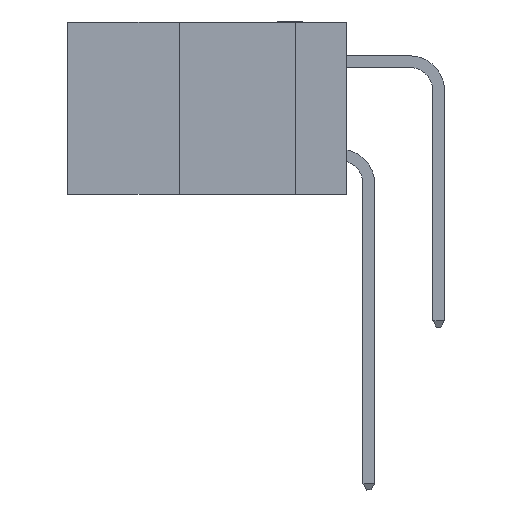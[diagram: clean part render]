
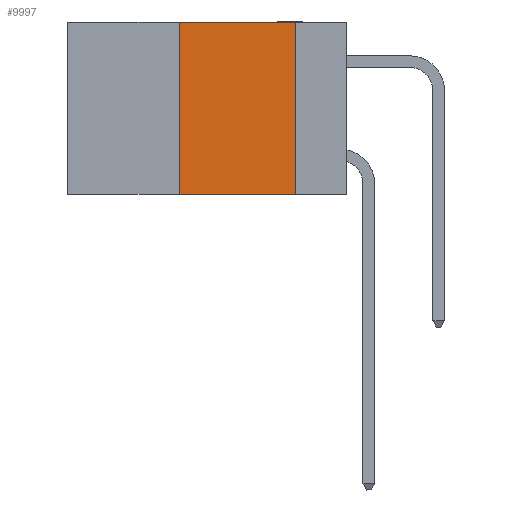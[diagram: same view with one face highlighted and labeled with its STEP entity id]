
A CAD part, left-side view. The second image highlights one B-rep face of the part: STEP entity #9997.
In plain terms, the highlighted planar face has unit normal (-1, 0, 0).
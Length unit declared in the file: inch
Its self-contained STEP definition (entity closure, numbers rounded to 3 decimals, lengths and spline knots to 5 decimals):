
#238 = FACE_OUTER_BOUND ( 'NONE', #1158, .T. ) ;
#518 = LINE ( 'NONE', #21421, #9261 ) ;
#585 = PLANE ( 'NONE',  #2373 ) ;
#899 = VECTOR ( 'NONE', #1618, 39.37008 ) ;
#1158 = EDGE_LOOP ( 'NONE', ( #18078, #10498, #21211, #17680 ) ) ;
#1618 = DIRECTION ( 'NONE',  ( 0., -1., 0. ) ) ;
#2373 = AXIS2_PLACEMENT_3D ( 'NONE', #12823, #14560, #4169 ) ;
#3454 = CARTESIAN_POINT ( 'NONE',  ( 0., 0.11, -0.37 ) ) ;
#3649 = VECTOR ( 'NONE', #14049, 39.37008 ) ;
#4169 = DIRECTION ( 'NONE',  ( 0., 0., -1. ) ) ;
#7463 = EDGE_CURVE ( 'NONE', #20679, #8522, #8081, .T. ) ;
#8081 = LINE ( 'NONE', #21353, #21289 ) ;
#8522 = VERTEX_POINT ( 'NONE', #3454 ) ;
#9073 = VERTEX_POINT ( 'NONE', #15743 ) ;
#9261 = VECTOR ( 'NONE', #11274, 39.37008 ) ;
#9997 = ADVANCED_FACE ( 'NONE', ( #238 ), #585, .F. ) ;
#10498 = ORIENTED_EDGE ( 'NONE', *, *, #18647, .F. ) ;
#11274 = DIRECTION ( 'NONE',  ( 0., 0., -1. ) ) ;
#11620 = VERTEX_POINT ( 'NONE', #16867 ) ;
#12285 = CARTESIAN_POINT ( 'NONE',  ( 0., 0.36, 0. ) ) ;
#12823 = CARTESIAN_POINT ( 'NONE',  ( 0., 0.6, 0. ) ) ;
#12903 = LINE ( 'NONE', #12285, #3649 ) ;
#14049 = DIRECTION ( 'NONE',  ( 0., 0., 1. ) ) ;
#14560 = DIRECTION ( 'NONE',  ( 1., 0., 0. ) ) ;
#14611 = DIRECTION ( 'NONE',  ( 0., -1., 0. ) ) ;
#14820 = LINE ( 'NONE', #22279, #899 ) ;
#15113 = EDGE_CURVE ( 'NONE', #11620, #8522, #518, .T. ) ;
#15743 = CARTESIAN_POINT ( 'NONE',  ( 0., 0.36, 0. ) ) ;
#16021 = CARTESIAN_POINT ( 'NONE',  ( 0., 0.36, -0.37 ) ) ;
#16867 = CARTESIAN_POINT ( 'NONE',  ( 0., 0.11, 0. ) ) ;
#17680 = ORIENTED_EDGE ( 'NONE', *, *, #7463, .T. ) ;
#18078 = ORIENTED_EDGE ( 'NONE', *, *, #15113, .F. ) ;
#18647 = EDGE_CURVE ( 'NONE', #9073, #11620, #14820, .T. ) ;
#19995 = EDGE_CURVE ( 'NONE', #20679, #9073, #12903, .T. ) ;
#20679 = VERTEX_POINT ( 'NONE', #16021 ) ;
#21211 = ORIENTED_EDGE ( 'NONE', *, *, #19995, .F. ) ;
#21289 = VECTOR ( 'NONE', #14611, 39.37008 ) ;
#21353 = CARTESIAN_POINT ( 'NONE',  ( 0., 0.6, -0.37 ) ) ;
#21421 = CARTESIAN_POINT ( 'NONE',  ( 0., 0.11, 0. ) ) ;
#22279 = CARTESIAN_POINT ( 'NONE',  ( 0., 0.6, 0. ) ) ;
